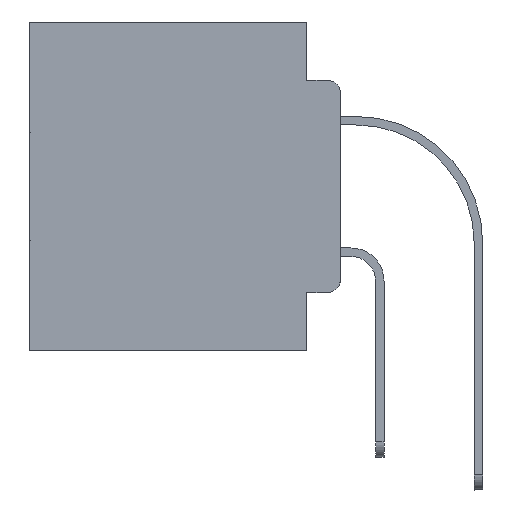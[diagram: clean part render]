
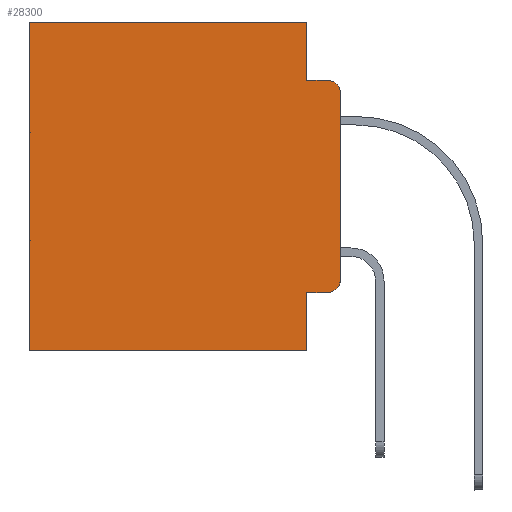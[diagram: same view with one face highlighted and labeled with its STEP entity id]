
A CAD part, left-side view. The second image highlights one B-rep face of the part: STEP entity #28300.
In plain terms, the highlighted planar face has unit normal (-1, 0, 0).
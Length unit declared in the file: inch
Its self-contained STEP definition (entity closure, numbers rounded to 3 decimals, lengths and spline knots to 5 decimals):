
#223 = DIRECTION ( 'NONE',  ( -1., 0., 0. ) ) ;
#529 = VERTEX_POINT ( 'NONE', #29756 ) ;
#1904 = VERTEX_POINT ( 'NONE', #26186 ) ;
#2059 = ORIENTED_EDGE ( 'NONE', *, *, #17964, .F. ) ;
#2555 = VECTOR ( 'NONE', #22335, 39.37008 ) ;
#2599 = EDGE_CURVE ( 'NONE', #1904, #28425, #5280, .T. ) ;
#2725 = EDGE_CURVE ( 'NONE', #19549, #22169, #10383, .T. ) ;
#2994 = ORIENTED_EDGE ( 'NONE', *, *, #28076, .T. ) ;
#3466 = VECTOR ( 'NONE', #20857, 39.37008 ) ;
#3569 = ORIENTED_EDGE ( 'NONE', *, *, #9778, .T. ) ;
#4863 = CARTESIAN_POINT ( 'NONE',  ( 0.298, 0.02, -0.1085 ) ) ;
#5280 = LINE ( 'NONE', #7059, #25423 ) ;
#5995 = LINE ( 'NONE', #22831, #8539 ) ;
#6214 = CARTESIAN_POINT ( 'NONE',  ( 0.298, 0.051, 0. ) ) ;
#6325 = ORIENTED_EDGE ( 'NONE', *, *, #17177, .F. ) ;
#6599 = ORIENTED_EDGE ( 'NONE', *, *, #29076, .F. ) ;
#7059 = CARTESIAN_POINT ( 'NONE',  ( 0.298, 0.051, -0.0885 ) ) ;
#7605 = DIRECTION ( 'NONE',  ( 1., 0., 0. ) ) ;
#8052 = VERTEX_POINT ( 'NONE', #20047 ) ;
#8066 = AXIS2_PLACEMENT_3D ( 'NONE', #4863, #223, #14618 ) ;
#8435 = LINE ( 'NONE', #6214, #22399 ) ;
#8438 = VECTOR ( 'NONE', #25158, 39.37008 ) ;
#8539 = VECTOR ( 'NONE', #15288, 39.37008 ) ;
#8550 = AXIS2_PLACEMENT_3D ( 'NONE', #12655, #17605, #30139 ) ;
#8582 = DIRECTION ( 'NONE',  ( 0., -1., 0. ) ) ;
#9778 = EDGE_CURVE ( 'NONE', #22459, #29465, #20337, .T. ) ;
#10263 = ORIENTED_EDGE ( 'NONE', *, *, #12373, .T. ) ;
#10383 = LINE ( 'NONE', #15352, #8438 ) ;
#10592 = AXIS2_PLACEMENT_3D ( 'NONE', #29561, #7605, #14159 ) ;
#11293 = LINE ( 'NONE', #25743, #18251 ) ;
#12159 = CIRCLE ( 'NONE', #8066, 0.02 ) ;
#12373 = EDGE_CURVE ( 'NONE', #21145, #19549, #22024, .T. ) ;
#12655 = CARTESIAN_POINT ( 'NONE',  ( 0.298, 0.02, -0.3915 ) ) ;
#13632 = ORIENTED_EDGE ( 'NONE', *, *, #30763, .T. ) ;
#14159 = DIRECTION ( 'NONE',  ( 0., 0., -1. ) ) ;
#14449 = ORIENTED_EDGE ( 'NONE', *, *, #2599, .F. ) ;
#14618 = DIRECTION ( 'NONE',  ( 0., 0., -1. ) ) ;
#14852 = CARTESIAN_POINT ( 'NONE',  ( 0.298, 0.02, -0.4115 ) ) ;
#15288 = DIRECTION ( 'NONE',  ( 0., 0., -1. ) ) ;
#15352 = CARTESIAN_POINT ( 'NONE',  ( 0.298, 0.473, 0. ) ) ;
#15457 = CARTESIAN_POINT ( 'NONE',  ( 0.298, 0.051, 0. ) ) ;
#15502 = CARTESIAN_POINT ( 'NONE',  ( 0.298, 0.473, -0.5 ) ) ;
#16345 = CARTESIAN_POINT ( 'NONE',  ( 0.298, 0.051, 0. ) ) ;
#16823 = VERTEX_POINT ( 'NONE', #27679 ) ;
#17177 = EDGE_CURVE ( 'NONE', #16823, #29465, #5995, .T. ) ;
#17605 = DIRECTION ( 'NONE',  ( -1., 0., 0. ) ) ;
#17964 = EDGE_CURVE ( 'NONE', #21145, #1904, #8435, .T. ) ;
#18073 = EDGE_CURVE ( 'NONE', #8052, #22169, #20310, .T. ) ;
#18251 = VECTOR ( 'NONE', #8582, 39.37008 ) ;
#19549 = VERTEX_POINT ( 'NONE', #28952 ) ;
#19793 = ORIENTED_EDGE ( 'NONE', *, *, #18073, .F. ) ;
#20047 = CARTESIAN_POINT ( 'NONE',  ( 0.298, 0.051, -0.5 ) ) ;
#20066 = EDGE_LOOP ( 'NONE', ( #6325, #13632, #14449, #2059, #10263, #22291, #19793, #6599, #2994, #3569 ) ) ;
#20310 = LINE ( 'NONE', #25285, #26030 ) ;
#20337 = CIRCLE ( 'NONE', #8550, 0.02 ) ;
#20491 = CARTESIAN_POINT ( 'NONE',  ( 0.298, 0., -0.3915 ) ) ;
#20857 = DIRECTION ( 'NONE',  ( 0., 0., -1. ) ) ;
#21145 = VERTEX_POINT ( 'NONE', #15457 ) ;
#22024 = LINE ( 'NONE', #22167, #2555 ) ;
#22167 = CARTESIAN_POINT ( 'NONE',  ( 0.298, 0., 0. ) ) ;
#22169 = VERTEX_POINT ( 'NONE', #15502 ) ;
#22291 = ORIENTED_EDGE ( 'NONE', *, *, #2725, .T. ) ;
#22335 = DIRECTION ( 'NONE',  ( 0., 1., 0. ) ) ;
#22399 = VECTOR ( 'NONE', #30106, 39.37008 ) ;
#22459 = VERTEX_POINT ( 'NONE', #14852 ) ;
#22831 = CARTESIAN_POINT ( 'NONE',  ( 0.298, 0., 0. ) ) ;
#24376 = DIRECTION ( 'NONE',  ( 0., -1., 0. ) ) ;
#25158 = DIRECTION ( 'NONE',  ( 0., 0., -1. ) ) ;
#25285 = CARTESIAN_POINT ( 'NONE',  ( 0.298, 0., -0.5 ) ) ;
#25423 = VECTOR ( 'NONE', #24376, 39.37008 ) ;
#25457 = DIRECTION ( 'NONE',  ( 0., 1., 0. ) ) ;
#25743 = CARTESIAN_POINT ( 'NONE',  ( 0.298, 0.051, -0.4115 ) ) ;
#26030 = VECTOR ( 'NONE', #25457, 39.37008 ) ;
#26186 = CARTESIAN_POINT ( 'NONE',  ( 0.298, 0.051, -0.0885 ) ) ;
#26679 = PLANE ( 'NONE',  #10592 ) ;
#27466 = CARTESIAN_POINT ( 'NONE',  ( 0.298, 0.02, -0.0885 ) ) ;
#27679 = CARTESIAN_POINT ( 'NONE',  ( 0.298, 0., -0.1085 ) ) ;
#28076 = EDGE_CURVE ( 'NONE', #529, #22459, #11293, .T. ) ;
#28300 = ADVANCED_FACE ( 'NONE', ( #28905 ), #26679, .F. ) ;
#28425 = VERTEX_POINT ( 'NONE', #27466 ) ;
#28905 = FACE_OUTER_BOUND ( 'NONE', #20066, .T. ) ;
#28952 = CARTESIAN_POINT ( 'NONE',  ( 0.298, 0.473, 0. ) ) ;
#29076 = EDGE_CURVE ( 'NONE', #529, #8052, #30799, .T. ) ;
#29465 = VERTEX_POINT ( 'NONE', #20491 ) ;
#29561 = CARTESIAN_POINT ( 'NONE',  ( 0.298, 0., 0. ) ) ;
#29756 = CARTESIAN_POINT ( 'NONE',  ( 0.298, 0.051, -0.4115 ) ) ;
#30106 = DIRECTION ( 'NONE',  ( 0., 0., -1. ) ) ;
#30139 = DIRECTION ( 'NONE',  ( 0., 0., -1. ) ) ;
#30763 = EDGE_CURVE ( 'NONE', #16823, #28425, #12159, .T. ) ;
#30799 = LINE ( 'NONE', #16345, #3466 ) ;
